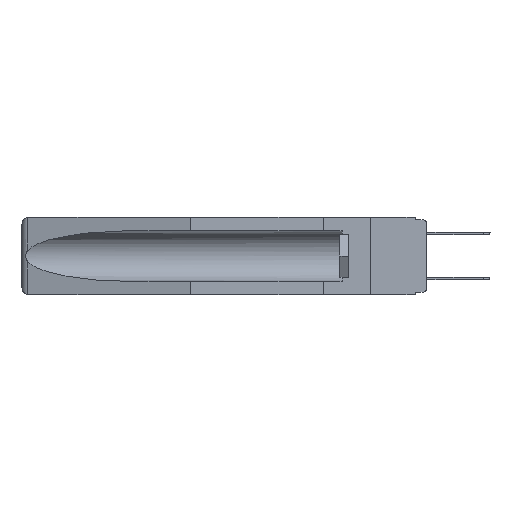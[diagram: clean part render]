
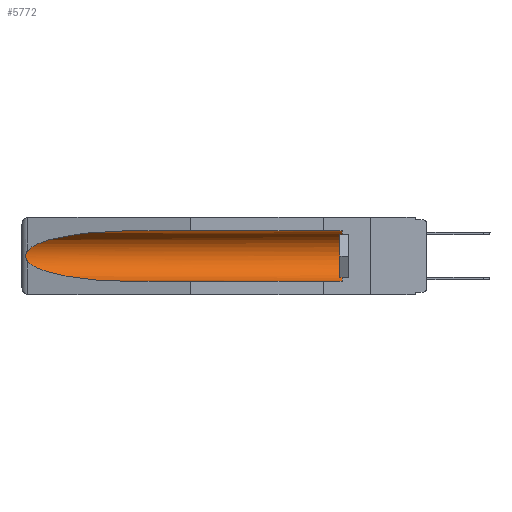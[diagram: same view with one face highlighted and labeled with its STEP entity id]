
A CAD part, left-side view. The second image highlights one B-rep face of the part: STEP entity #5772.
In plain terms, the highlighted cylindrical face has radius 2.857 mm (diameter 5.715 mm), a partial arc.
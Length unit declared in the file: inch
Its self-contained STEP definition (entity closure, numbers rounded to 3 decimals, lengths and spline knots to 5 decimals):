
#208 = EDGE_CURVE ( 'NONE', #12022, #6118, #1682, .T. ) ;
#829 = CARTESIAN_POINT ( 'NONE',  ( 0.155, -0.30754, -0.284 ) ) ;
#951 = CARTESIAN_POINT ( 'NONE',  ( 0.2675, 1.53308, -0.17534 ) ) ;
#1003 = VERTEX_POINT ( 'NONE', #11896 ) ;
#1212 = ORIENTED_EDGE ( 'NONE', *, *, #5108, .T. ) ;
#1287 = CYLINDRICAL_SURFACE ( 'NONE', #11497, 0.1125 ) ;
#1403 = VECTOR ( 'NONE', #9070, 39.37008 ) ;
#1682 =( BOUNDED_CURVE ( )  B_SPLINE_CURVE ( 3, ( #16712, #5845, #3353, #9845 ),
 .UNSPECIFIED., .F., .T. ) 
 B_SPLINE_CURVE_WITH_KNOTS ( ( 4, 4 ),
 ( 0.1948, 1.5708 ),
 .UNSPECIFIED. ) 
 CURVE ( )  GEOMETRIC_REPRESENTATION_ITEM ( )  RATIONAL_B_SPLINE_CURVE ( ( 1., 0.848, 0.848, 1. ) ) 
 REPRESENTATION_ITEM ( '' )  );
#1694 = VERTEX_POINT ( 'NONE', #16996 ) ;
#1932 = DIRECTION ( 'NONE',  ( 0., 0., 1. ) ) ;
#2040 = EDGE_LOOP ( 'NONE', ( #4811, #3092, #2441, #10276, #1212, #3144 ) ) ;
#2441 = ORIENTED_EDGE ( 'NONE', *, *, #208, .T. ) ;
#3092 = ORIENTED_EDGE ( 'NONE', *, *, #10739, .T. ) ;
#3144 = ORIENTED_EDGE ( 'NONE', *, *, #15475, .T. ) ;
#3182 = VECTOR ( 'NONE', #15229, 39.37008 ) ;
#3353 = CARTESIAN_POINT ( 'NONE',  ( 0.21114, 1.30732, -0.284 ) ) ;
#3435 = CARTESIAN_POINT ( 'NONE',  ( 0.26655, 1.53094, -0.18657 ) ) ;
#4670 = VERTEX_POINT ( 'NONE', #11989 ) ;
#4811 = ORIENTED_EDGE ( 'NONE', *, *, #13849, .T. ) ;
#5108 = EDGE_CURVE ( 'NONE', #1003, #12662, #16305, .T. ) ;
#5772 = ADVANCED_FACE ( 'NONE', ( #16425 ), #1287, .F. ) ;
#5845 = CARTESIAN_POINT ( 'NONE',  ( 0.25451, 1.48313, -0.24835 ) ) ;
#5934 = CARTESIAN_POINT ( 'NONE',  ( 0.155, -0.30754, -0.059 ) ) ;
#6118 = VERTEX_POINT ( 'NONE', #8900 ) ;
#6260 = CARTESIAN_POINT ( 'NONE',  ( 0.26654, 1.53092, -0.15636 ) ) ;
#6309 = LINE ( 'NONE', #829, #1403 ) ;
#6532 = CARTESIAN_POINT ( 'NONE',  ( 0.26537, 1.52718, -0.19328 ) ) ;
#6686 = CARTESIAN_POINT ( 'NONE',  ( 0.155, 0.126, -0.059 ) ) ;
#7049 = CARTESIAN_POINT ( 'NONE',  ( 0.155, -0.30754, -0.1715 ) ) ;
#7193 = CARTESIAN_POINT ( 'NONE',  ( 0.26537, 1.52718, -0.19328 ) ) ;
#7521 = CARTESIAN_POINT ( 'NONE',  ( 0.2675, 1.53308, -0.16763 ) ) ;
#7699 = CARTESIAN_POINT ( 'NONE',  ( 0.26597, 1.5296, -0.19026 ) ) ;
#7818 =( BOUNDED_CURVE ( )  B_SPLINE_CURVE ( 3, ( #13089, #10494, #11581, #15953 ),
 .UNSPECIFIED., .F., .T. ) 
 B_SPLINE_CURVE_WITH_KNOTS ( ( 4, 4 ),
 ( 4.71239, 6.08839 ),
 .UNSPECIFIED. ) 
 CURVE ( )  GEOMETRIC_REPRESENTATION_ITEM ( )  RATIONAL_B_SPLINE_CURVE ( ( 1., 0.848, 0.848, 1. ) ) 
 REPRESENTATION_ITEM ( '' )  );
#7874 = CARTESIAN_POINT ( 'NONE',  ( 0.2673, 1.53269, -0.17917 ) ) ;
#8592 = AXIS2_PLACEMENT_3D ( 'NONE', #8774, #14146, #1932 ) ;
#8769 = LINE ( 'NONE', #5934, #3182 ) ;
#8774 = CARTESIAN_POINT ( 'NONE',  ( 0.155, 0.126, -0.1715 ) ) ;
#8900 = CARTESIAN_POINT ( 'NONE',  ( 0.155, 1.07973, -0.284 ) ) ;
#9070 = DIRECTION ( 'NONE',  ( 0., 1., 0. ) ) ;
#9845 = CARTESIAN_POINT ( 'NONE',  ( 0.155, 1.07973, -0.284 ) ) ;
#10276 = ORIENTED_EDGE ( 'NONE', *, *, #12874, .F. ) ;
#10494 = CARTESIAN_POINT ( 'NONE',  ( 0.21114, 1.30732, -0.059 ) ) ;
#10547 = CARTESIAN_POINT ( 'NONE',  ( 0.2673, 1.5327, -0.16383 ) ) ;
#10739 = EDGE_CURVE ( 'NONE', #4670, #12022, #15216, .T. ) ;
#11497 = AXIS2_PLACEMENT_3D ( 'NONE', #7049, #17491, #12416 ) ;
#11581 = CARTESIAN_POINT ( 'NONE',  ( 0.25451, 1.48313, -0.09465 ) ) ;
#11896 = CARTESIAN_POINT ( 'NONE',  ( 0.155, 0.126, -0.284 ) ) ;
#11989 = CARTESIAN_POINT ( 'NONE',  ( 0.26537, 1.52718, -0.14972 ) ) ;
#12022 = VERTEX_POINT ( 'NONE', #7193 ) ;
#12416 = DIRECTION ( 'NONE',  ( 0., 0., 1. ) ) ;
#12662 = VERTEX_POINT ( 'NONE', #6686 ) ;
#12874 = EDGE_CURVE ( 'NONE', #1003, #6118, #6309, .T. ) ;
#13089 = CARTESIAN_POINT ( 'NONE',  ( 0.155, 1.07973, -0.059 ) ) ;
#13148 = CARTESIAN_POINT ( 'NONE',  ( 0.26537, 1.52718, -0.14972 ) ) ;
#13849 = EDGE_CURVE ( 'NONE', #1694, #4670, #7818, .T. ) ;
#14146 = DIRECTION ( 'NONE',  ( 0., -1., 0. ) ) ;
#15216 = B_SPLINE_CURVE_WITH_KNOTS ( 'NONE', 3,
 ( #13148, #15929, #6260, #10547, #7521, #951, #7874, #3435, #7699, #6532 ),
 .UNSPECIFIED., .F., .F.,
 ( 4, 2, 2, 2, 4 ),
 ( 0., 0.00029, 0.00058, 0.00087, 0.00117 ),
 .UNSPECIFIED. ) ;
#15229 = DIRECTION ( 'NONE',  ( 0., 1., 0. ) ) ;
#15475 = EDGE_CURVE ( 'NONE', #12662, #1694, #8769, .T. ) ;
#15929 = CARTESIAN_POINT ( 'NONE',  ( 0.26597, 1.52961, -0.15275 ) ) ;
#15953 = CARTESIAN_POINT ( 'NONE',  ( 0.26537, 1.52718, -0.14972 ) ) ;
#16305 = CIRCLE ( 'NONE', #8592, 0.1125 ) ;
#16425 = FACE_OUTER_BOUND ( 'NONE', #2040, .T. ) ;
#16712 = CARTESIAN_POINT ( 'NONE',  ( 0.26537, 1.52718, -0.19328 ) ) ;
#16996 = CARTESIAN_POINT ( 'NONE',  ( 0.155, 1.07973, -0.059 ) ) ;
#17491 = DIRECTION ( 'NONE',  ( 0., 1., 0. ) ) ;
